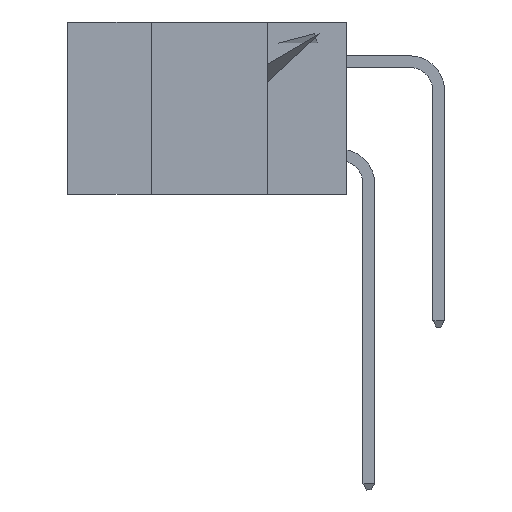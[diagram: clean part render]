
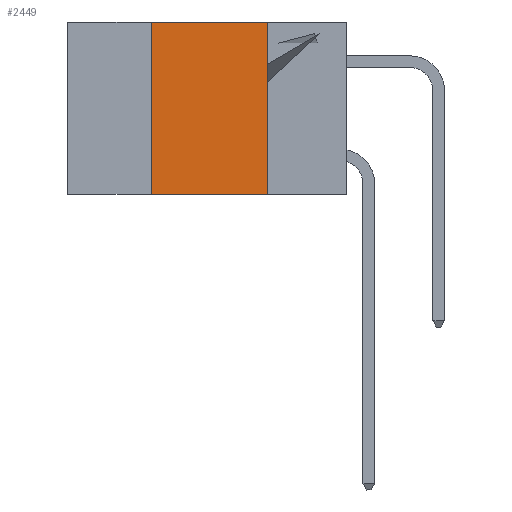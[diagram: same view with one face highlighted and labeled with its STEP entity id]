
A CAD part, left-side view. The second image highlights one B-rep face of the part: STEP entity #2449.
In plain terms, the highlighted planar face has unit normal (-1, 0, 0).
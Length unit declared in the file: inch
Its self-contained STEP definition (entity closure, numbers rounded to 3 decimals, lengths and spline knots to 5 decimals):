
#367 = LINE ( 'NONE', #4186, #3397 ) ;
#1055 = CARTESIAN_POINT ( 'NONE',  ( 0., 0.42, -0.37 ) ) ;
#1586 = LINE ( 'NONE', #10418, #12534 ) ;
#2003 = CARTESIAN_POINT ( 'NONE',  ( 0., 0.42, 0. ) ) ;
#2166 = CARTESIAN_POINT ( 'NONE',  ( 0., 0.17, -0.37 ) ) ;
#2309 = EDGE_CURVE ( 'NONE', #9819, #12339, #1586, .T. ) ;
#2449 = ADVANCED_FACE ( 'NONE', ( #8160 ), #8951, .F. ) ;
#2514 = EDGE_LOOP ( 'NONE', ( #5224, #5302, #5311, #5423 ) ) ;
#3014 = EDGE_CURVE ( 'NONE', #12339, #5753, #8306, .T. ) ;
#3260 = AXIS2_PLACEMENT_3D ( 'NONE', #9040, #8935, #8898 ) ;
#3293 = DIRECTION ( 'NONE',  ( 0., 0., -1. ) ) ;
#3311 = CARTESIAN_POINT ( 'NONE',  ( 0., 0.17, 0. ) ) ;
#3397 = VECTOR ( 'NONE', #7340, 39.37008 ) ;
#3796 = CARTESIAN_POINT ( 'NONE',  ( 0., 0.6, -0.37 ) ) ;
#4186 = CARTESIAN_POINT ( 'NONE',  ( 0., 0.42, 0. ) ) ;
#5224 = ORIENTED_EDGE ( 'NONE', *, *, #3014, .F. ) ;
#5302 = ORIENTED_EDGE ( 'NONE', *, *, #2309, .F. ) ;
#5311 = ORIENTED_EDGE ( 'NONE', *, *, #12361, .F. ) ;
#5423 = ORIENTED_EDGE ( 'NONE', *, *, #12856, .T. ) ;
#5545 = VECTOR ( 'NONE', #3293, 39.37008 ) ;
#5753 = VERTEX_POINT ( 'NONE', #2166 ) ;
#7340 = DIRECTION ( 'NONE',  ( 0., 0., 1. ) ) ;
#8160 = FACE_OUTER_BOUND ( 'NONE', #2514, .T. ) ;
#8306 = LINE ( 'NONE', #3311, #5545 ) ;
#8898 = DIRECTION ( 'NONE',  ( 0., 0., -1. ) ) ;
#8935 = DIRECTION ( 'NONE',  ( 1., 0., 0. ) ) ;
#8951 = PLANE ( 'NONE',  #3260 ) ;
#9040 = CARTESIAN_POINT ( 'NONE',  ( 0., 0.6, 0. ) ) ;
#9281 = LINE ( 'NONE', #3796, #12404 ) ;
#9819 = VERTEX_POINT ( 'NONE', #2003 ) ;
#10342 = DIRECTION ( 'NONE',  ( 0., -1., 0. ) ) ;
#10418 = CARTESIAN_POINT ( 'NONE',  ( 0., 0.6, 0. ) ) ;
#10421 = CARTESIAN_POINT ( 'NONE',  ( 0., 0.17, 0. ) ) ;
#12339 = VERTEX_POINT ( 'NONE', #10421 ) ;
#12361 = EDGE_CURVE ( 'NONE', #12552, #9819, #367, .T. ) ;
#12404 = VECTOR ( 'NONE', #13157, 39.37008 ) ;
#12534 = VECTOR ( 'NONE', #10342, 39.37008 ) ;
#12552 = VERTEX_POINT ( 'NONE', #1055 ) ;
#12856 = EDGE_CURVE ( 'NONE', #12552, #5753, #9281, .T. ) ;
#13157 = DIRECTION ( 'NONE',  ( 0., -1., 0. ) ) ;
